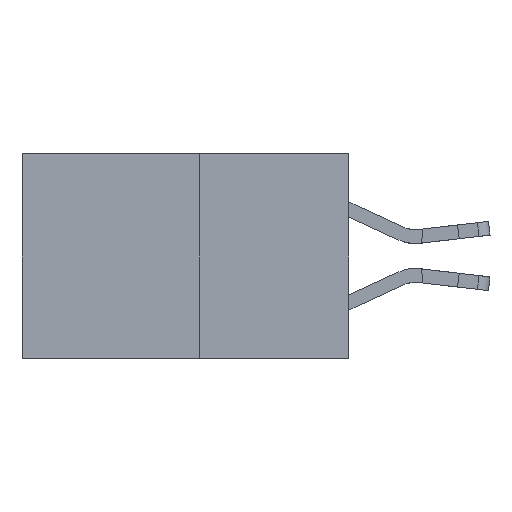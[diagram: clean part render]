
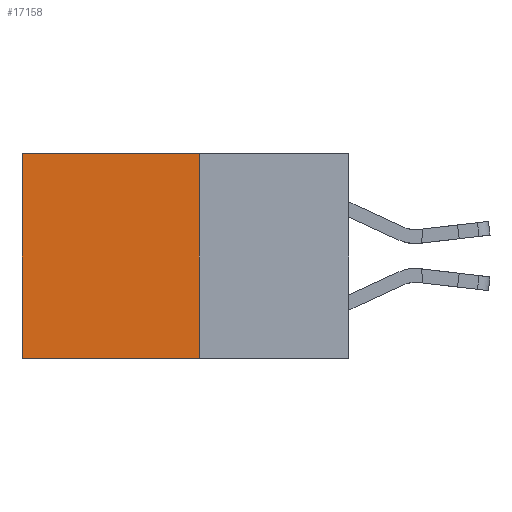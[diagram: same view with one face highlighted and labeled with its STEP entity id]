
A CAD part, left-side view. The second image highlights one B-rep face of the part: STEP entity #17158.
In plain terms, the highlighted planar face has unit normal (-1, 0, 0).
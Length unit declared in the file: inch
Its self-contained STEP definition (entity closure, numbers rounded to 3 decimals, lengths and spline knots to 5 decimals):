
#406 = EDGE_CURVE ( 'NONE', #7048, #11012, #18282, .T. ) ;
#1010 = CARTESIAN_POINT ( 'NONE',  ( 0.277, 0.27, -0.37 ) ) ;
#1212 = DIRECTION ( 'NONE',  ( 0., 1., 0. ) ) ;
#3314 = DIRECTION ( 'NONE',  ( 0., 0., -1. ) ) ;
#3508 = CARTESIAN_POINT ( 'NONE',  ( 0.277, 0.27, 0. ) ) ;
#3642 = CARTESIAN_POINT ( 'NONE',  ( 0.277, 0.59, -0.37 ) ) ;
#3996 = VECTOR ( 'NONE', #1212, 39.37008 ) ;
#4902 = CARTESIAN_POINT ( 'NONE',  ( 0.277, 0.27, -0.37 ) ) ;
#5968 = CARTESIAN_POINT ( 'NONE',  ( 0.277, 0.27, 0. ) ) ;
#7048 = VERTEX_POINT ( 'NONE', #16617 ) ;
#8523 = CARTESIAN_POINT ( 'NONE',  ( 0.277, 0.59, -0.37 ) ) ;
#8962 = ORIENTED_EDGE ( 'NONE', *, *, #406, .T. ) ;
#9299 = EDGE_CURVE ( 'NONE', #13155, #11012, #24233, .T. ) ;
#9971 = ORIENTED_EDGE ( 'NONE', *, *, #9299, .F. ) ;
#11012 = VERTEX_POINT ( 'NONE', #3642 ) ;
#12120 = DIRECTION ( 'NONE',  ( 0., 0., -1. ) ) ;
#12252 = VECTOR ( 'NONE', #12120, 39.37008 ) ;
#12420 = PLANE ( 'NONE',  #26846 ) ;
#12799 = EDGE_CURVE ( 'NONE', #27224, #13155, #19399, .T. ) ;
#12883 = VECTOR ( 'NONE', #24066, 39.37008 ) ;
#13155 = VERTEX_POINT ( 'NONE', #15345 ) ;
#13396 = VECTOR ( 'NONE', #18697, 39.37008 ) ;
#15345 = CARTESIAN_POINT ( 'NONE',  ( 0.277, 0.27, -0.37 ) ) ;
#15466 = FACE_OUTER_BOUND ( 'NONE', #17292, .T. ) ;
#16256 = LINE ( 'NONE', #3508, #3996 ) ;
#16617 = CARTESIAN_POINT ( 'NONE',  ( 0.277, 0.59, 0. ) ) ;
#17101 = DIRECTION ( 'NONE',  ( 1., 0., 0. ) ) ;
#17158 = ADVANCED_FACE ( 'NONE', ( #15466 ), #12420, .F. ) ;
#17292 = EDGE_LOOP ( 'NONE', ( #8962, #9971, #25249, #24968 ) ) ;
#18282 = LINE ( 'NONE', #8523, #12252 ) ;
#18697 = DIRECTION ( 'NONE',  ( 0., 0., -1. ) ) ;
#19399 = LINE ( 'NONE', #4902, #13396 ) ;
#24066 = DIRECTION ( 'NONE',  ( 0., 1., 0. ) ) ;
#24233 = LINE ( 'NONE', #24250, #12883 ) ;
#24250 = CARTESIAN_POINT ( 'NONE',  ( 0.277, 0.27, -0.37 ) ) ;
#24968 = ORIENTED_EDGE ( 'NONE', *, *, #27195, .T. ) ;
#25249 = ORIENTED_EDGE ( 'NONE', *, *, #12799, .F. ) ;
#26846 = AXIS2_PLACEMENT_3D ( 'NONE', #1010, #17101, #3314 ) ;
#27195 = EDGE_CURVE ( 'NONE', #27224, #7048, #16256, .T. ) ;
#27224 = VERTEX_POINT ( 'NONE', #5968 ) ;
